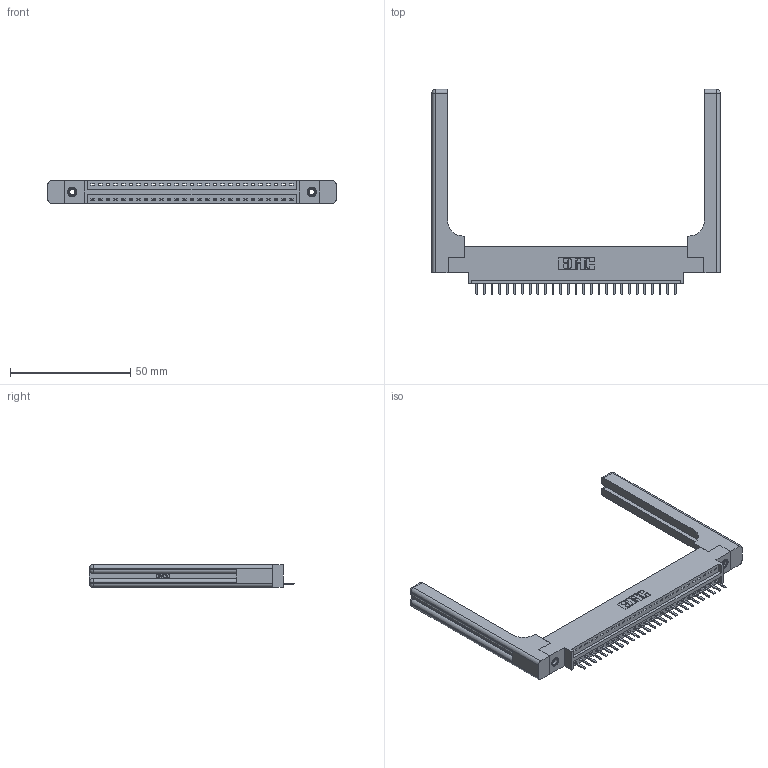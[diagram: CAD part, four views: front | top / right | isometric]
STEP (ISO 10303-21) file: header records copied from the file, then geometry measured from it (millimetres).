
FILE_DESCRIPTION (( 'STEP AP203' ), '1' );
FILE_NAME ('346-027-520-658.STEP', '2022-05-06T04:11:22', ( '' ), ( '' ), 'SwSTEP 2.0', 'SolidWorks 2020', '' );
FILE_SCHEMA (( 'CONFIG_CONTROL_DESIGN' ));
Length unit declared in the file: inch
Products named in the file (5): 345-250-001_345-250-001-102; 346-027-520-658; 345-292-001_345-293-120; 346 Part_0.170 Offset - 0.156 Dia-TH; 346-220-058_345-220-058
Assembly tree (32 placements, depth 2):
  346-027-520-658
    346 Part_0.170 Offset - 0.156 Dia-TH
    345-292-001_345-293-120  x27
    345-250-001_345-250-001-102  x2
    346-220-058_345-220-058  x2
Bounding box: 119.79 x 85.29 x 9.4 mm (x, y, z)
Volume: 18630.9 mm3; surface area: 18830.2 mm2
Topology: 32 solids, 32 shells, 2070 faces, 6011 edges, 3914 vertices
Faces by surface type: plane 1376, cylinder 634, bspline 36, cone 12, sphere 8, torus 4
Entity records: 24620 total; most frequent: CARTESIAN_POINT 5220, ORIENTED_EDGE 3964, DIRECTION 3540, EDGE_CURVE 1982, LINE 1646, VECTOR 1646, VERTEX_POINT 1310, AXIS2_PLACEMENT_3D 947
